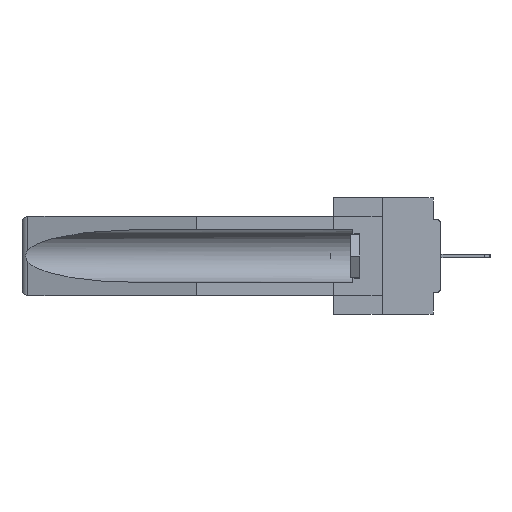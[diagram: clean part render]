
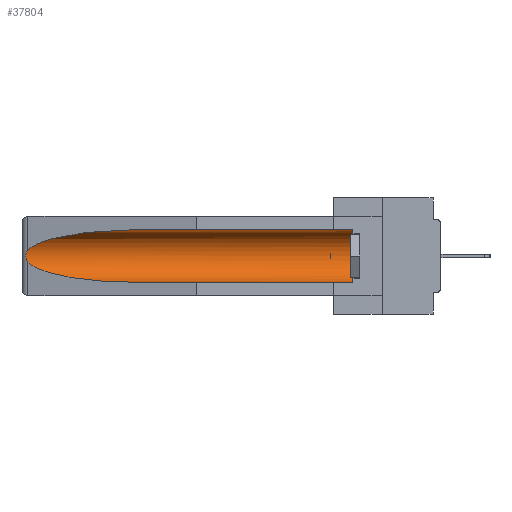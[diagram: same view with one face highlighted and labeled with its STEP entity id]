
A CAD part, left-side view. The second image highlights one B-rep face of the part: STEP entity #37804.
In plain terms, the highlighted cylindrical face has radius 2.857 mm (diameter 5.715 mm), a partial arc.
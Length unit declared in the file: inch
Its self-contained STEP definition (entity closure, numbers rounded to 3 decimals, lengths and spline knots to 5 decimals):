
#178 = EDGE_CURVE ( 'NONE', #4108, #23116, #3957, .T. ) ;
#444 = DIRECTION ( 'NONE',  ( 0., 0., 1. ) ) ;
#508 = LINE ( 'NONE', #14671, #11768 ) ;
#2418 = CARTESIAN_POINT ( 'NONE',  ( 0.26537, 1.52718, -0.14972 ) ) ;
#3604 = DIRECTION ( 'NONE',  ( 0., -1., 0. ) ) ;
#3957 =( BOUNDED_CURVE ( )  B_SPLINE_CURVE ( 3, ( #11715, #38400, #41561, #2418 ),
 .UNSPECIFIED., .F., .F. ) 
 B_SPLINE_CURVE_WITH_KNOTS ( ( 4, 4 ),
 ( 4.71239, 6.08839 ),
 .UNSPECIFIED. ) 
 CURVE ( )  GEOMETRIC_REPRESENTATION_ITEM ( )  RATIONAL_B_SPLINE_CURVE ( ( 1., 0.848, 0.848, 1. ) ) 
 REPRESENTATION_ITEM ( '' )  );
#4108 = VERTEX_POINT ( 'NONE', #22666 ) ;
#4185 = DIRECTION ( 'NONE',  ( 0., 1., 0. ) ) ;
#5209 = CARTESIAN_POINT ( 'NONE',  ( 0.26597, 1.5296, -0.19026 ) ) ;
#9092 = VERTEX_POINT ( 'NONE', #33936 ) ;
#10333 = CARTESIAN_POINT ( 'NONE',  ( 0.155, -0.30754, -0.1715 ) ) ;
#11352 = CARTESIAN_POINT ( 'NONE',  ( 0.26537, 1.52718, -0.14972 ) ) ;
#11569 =( BOUNDED_CURVE ( )  B_SPLINE_CURVE ( 3, ( #12954, #26200, #19524, #16490 ),
 .UNSPECIFIED., .F., .F. ) 
 B_SPLINE_CURVE_WITH_KNOTS ( ( 4, 4 ),
 ( 0.1948, 1.5708 ),
 .UNSPECIFIED. ) 
 CURVE ( )  GEOMETRIC_REPRESENTATION_ITEM ( )  RATIONAL_B_SPLINE_CURVE ( ( 1., 0.848, 0.848, 1. ) ) 
 REPRESENTATION_ITEM ( '' )  );
#11715 = CARTESIAN_POINT ( 'NONE',  ( 0.155, 1.07973, -0.059 ) ) ;
#11768 = VECTOR ( 'NONE', #34358, 39.37008 ) ;
#12621 = CARTESIAN_POINT ( 'NONE',  ( 0.26537, 1.52718, -0.14972 ) ) ;
#12677 = CARTESIAN_POINT ( 'NONE',  ( 0.155, 1.07973, -0.284 ) ) ;
#12929 = AXIS2_PLACEMENT_3D ( 'NONE', #20022, #3604, #444 ) ;
#12954 = CARTESIAN_POINT ( 'NONE',  ( 0.26537, 1.52718, -0.19328 ) ) ;
#14550 = CYLINDRICAL_SURFACE ( 'NONE', #28154, 0.1125 ) ;
#14617 = CARTESIAN_POINT ( 'NONE',  ( 0.2673, 1.53269, -0.17917 ) ) ;
#14671 = CARTESIAN_POINT ( 'NONE',  ( 0.155, -0.30754, -0.059 ) ) ;
#15508 = CARTESIAN_POINT ( 'NONE',  ( 0.26537, 1.52718, -0.19328 ) ) ;
#16490 = CARTESIAN_POINT ( 'NONE',  ( 0.155, 1.07973, -0.284 ) ) ;
#16832 = ORIENTED_EDGE ( 'NONE', *, *, #19279, .T. ) ;
#17888 = CARTESIAN_POINT ( 'NONE',  ( 0.26655, 1.53094, -0.18657 ) ) ;
#18139 = CIRCLE ( 'NONE', #12929, 0.1125 ) ;
#19279 = EDGE_CURVE ( 'NONE', #39074, #37124, #11569, .T. ) ;
#19524 = CARTESIAN_POINT ( 'NONE',  ( 0.21114, 1.30732, -0.284 ) ) ;
#19903 = DIRECTION ( 'NONE',  ( 0., 1., 0. ) ) ;
#20022 = CARTESIAN_POINT ( 'NONE',  ( 0.155, 0.126, -0.1715 ) ) ;
#21293 = ORIENTED_EDGE ( 'NONE', *, *, #28872, .T. ) ;
#22666 = CARTESIAN_POINT ( 'NONE',  ( 0.155, 1.07973, -0.059 ) ) ;
#22930 = EDGE_CURVE ( 'NONE', #23116, #39074, #35621, .T. ) ;
#23116 = VERTEX_POINT ( 'NONE', #12621 ) ;
#24171 = CARTESIAN_POINT ( 'NONE',  ( 0.2673, 1.5327, -0.16383 ) ) ;
#26200 = CARTESIAN_POINT ( 'NONE',  ( 0.25451, 1.48313, -0.24835 ) ) ;
#28154 = AXIS2_PLACEMENT_3D ( 'NONE', #10333, #4185, #36851 ) ;
#28872 = EDGE_CURVE ( 'NONE', #9092, #37667, #18139, .T. ) ;
#30609 = ORIENTED_EDGE ( 'NONE', *, *, #178, .T. ) ;
#31000 = VECTOR ( 'NONE', #19903, 39.37008 ) ;
#31283 = CARTESIAN_POINT ( 'NONE',  ( 0.26654, 1.53092, -0.15636 ) ) ;
#31890 = CARTESIAN_POINT ( 'NONE',  ( 0.155, -0.30754, -0.284 ) ) ;
#32288 = CARTESIAN_POINT ( 'NONE',  ( 0.155, 0.126, -0.059 ) ) ;
#33328 = ORIENTED_EDGE ( 'NONE', *, *, #33537, .T. ) ;
#33537 = EDGE_CURVE ( 'NONE', #37667, #4108, #508, .T. ) ;
#33835 = ORIENTED_EDGE ( 'NONE', *, *, #22930, .T. ) ;
#33936 = CARTESIAN_POINT ( 'NONE',  ( 0.155, 0.126, -0.284 ) ) ;
#34154 = CARTESIAN_POINT ( 'NONE',  ( 0.2675, 1.53308, -0.17534 ) ) ;
#34201 = EDGE_LOOP ( 'NONE', ( #30609, #33835, #16832, #38273, #21293, #33328 ) ) ;
#34294 = CARTESIAN_POINT ( 'NONE',  ( 0.2675, 1.53308, -0.16763 ) ) ;
#34358 = DIRECTION ( 'NONE',  ( 0., 1., 0. ) ) ;
#35621 = B_SPLINE_CURVE_WITH_KNOTS ( 'NONE', 3,
 ( #11352, #37745, #31283, #24171, #34294, #34154, #14617, #17888, #5209, #40741 ),
 .UNSPECIFIED., .F., .F.,
 ( 4, 2, 2, 2, 4 ),
 ( 0., 0.00029, 0.00058, 0.00087, 0.00117 ),
 .UNSPECIFIED. ) ;
#36661 = LINE ( 'NONE', #31890, #31000 ) ;
#36851 = DIRECTION ( 'NONE',  ( 0., 0., 1. ) ) ;
#37124 = VERTEX_POINT ( 'NONE', #12677 ) ;
#37667 = VERTEX_POINT ( 'NONE', #32288 ) ;
#37745 = CARTESIAN_POINT ( 'NONE',  ( 0.26597, 1.52961, -0.15275 ) ) ;
#37804 = ADVANCED_FACE ( 'NONE', ( #41119 ), #14550, .F. ) ;
#38273 = ORIENTED_EDGE ( 'NONE', *, *, #42331, .F. ) ;
#38400 = CARTESIAN_POINT ( 'NONE',  ( 0.21114, 1.30732, -0.059 ) ) ;
#39074 = VERTEX_POINT ( 'NONE', #15508 ) ;
#40741 = CARTESIAN_POINT ( 'NONE',  ( 0.26537, 1.52718, -0.19328 ) ) ;
#41119 = FACE_OUTER_BOUND ( 'NONE', #34201, .T. ) ;
#41561 = CARTESIAN_POINT ( 'NONE',  ( 0.25451, 1.48313, -0.09465 ) ) ;
#42331 = EDGE_CURVE ( 'NONE', #9092, #37124, #36661, .T. ) ;
